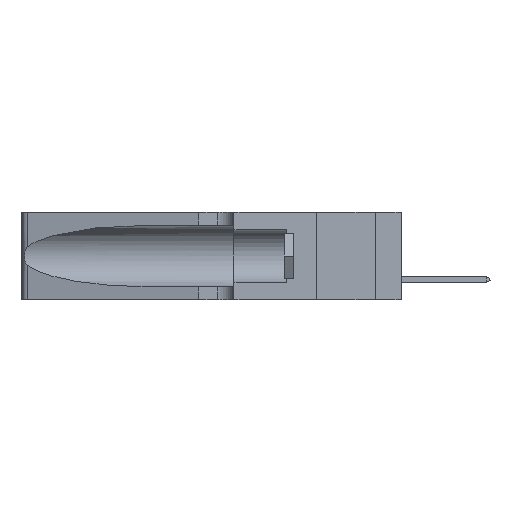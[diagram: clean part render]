
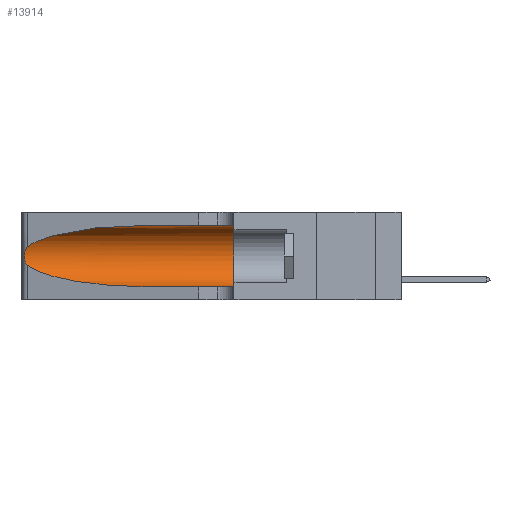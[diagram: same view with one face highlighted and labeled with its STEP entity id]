
A CAD part, left-side view. The second image highlights one B-rep face of the part: STEP entity #13914.
In plain terms, the highlighted cylindrical face has radius 3.308 mm (diameter 6.617 mm), a partial arc.
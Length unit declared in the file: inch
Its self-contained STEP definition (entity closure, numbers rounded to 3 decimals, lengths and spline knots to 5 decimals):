
#699 = DIRECTION ( 'NONE',  ( 0., -1., 0. ) ) ;
#1340 = CARTESIAN_POINT ( 'NONE',  ( 0.25487, 1.22718, 0.22369 ) ) ;
#1748 = ORIENTED_EDGE ( 'NONE', *, *, #21089, .T. ) ;
#2220 = VERTEX_POINT ( 'NONE', #32454 ) ;
#2355 = CARTESIAN_POINT ( 'NONE',  ( 0.1305, 1.61858, 0.05475 ) ) ;
#2359 = CARTESIAN_POINT ( 'NONE',  ( 0.26075, 1.23896, 0.19203 ) ) ;
#2430 = AXIS2_PLACEMENT_3D ( 'NONE', #25510, #30448, #20397 ) ;
#2759 = CARTESIAN_POINT ( 'NONE',  ( 0.1305, 1.61858, 0.31525 ) ) ;
#2851 = VECTOR ( 'NONE', #5037, 39.37008 ) ;
#3721 = EDGE_CURVE ( 'NONE', #10846, #26673, #28995, .T. ) ;
#3957 = DIRECTION ( 'NONE',  ( 0., 0., 1. ) ) ;
#4717 = CARTESIAN_POINT ( 'NONE',  ( 0.25787, 1.23484, 0.2124 ) ) ;
#5037 = DIRECTION ( 'NONE',  ( 0., -1., 0. ) ) ;
#5045 = CARTESIAN_POINT ( 'NONE',  ( 0.25789, 1.23486, 0.15765 ) ) ;
#6165 = CARTESIAN_POINT ( 'NONE',  ( 0.18966, 0.96281, 0.05475 ) ) ;
#7093 = CARTESIAN_POINT ( 'NONE',  ( 0.25487, 1.22718, 0.14631 ) ) ;
#7228 = EDGE_CURVE ( 'NONE', #19252, #17524, #25110, .T. ) ;
#7831 = EDGE_CURVE ( 'NONE', #2220, #19252, #24213, .T. ) ;
#8399 = CARTESIAN_POINT ( 'NONE',  ( 0.2373, 1.15595, 0.08982 ) ) ;
#8485 = CYLINDRICAL_SURFACE ( 'NONE', #2430, 0.13025 ) ;
#9844 = AXIS2_PLACEMENT_3D ( 'NONE', #29628, #32328, #3957 ) ;
#10044 =( BOUNDED_CURVE ( )  B_SPLINE_CURVE ( 3, ( #19012, #8399, #6165, #18335 ),
 .UNSPECIFIED., .F., .T. ) 
 B_SPLINE_CURVE_WITH_KNOTS ( ( 4, 4 ),
 ( 3.44316, 4.71239 ),
 .UNSPECIFIED. ) 
 CURVE ( )  GEOMETRIC_REPRESENTATION_ITEM ( )  RATIONAL_B_SPLINE_CURVE ( ( 1., 0.87, 0.87, 1. ) ) 
 REPRESENTATION_ITEM ( '' )  );
#10526 = CARTESIAN_POINT ( 'NONE',  ( 0.1305, 0.35, 0.05475 ) ) ;
#10846 = VERTEX_POINT ( 'NONE', #13500 ) ;
#11152 = ORIENTED_EDGE ( 'NONE', *, *, #7228, .F. ) ;
#12711 = CARTESIAN_POINT ( 'NONE',  ( 0.25854, 1.2359, 0.20912 ) ) ;
#13500 = CARTESIAN_POINT ( 'NONE',  ( 0.25487, 1.22718, 0.22369 ) ) ;
#13914 = ADVANCED_FACE ( 'NONE', ( #15770 ), #8485, .F. ) ;
#14806 = CARTESIAN_POINT ( 'NONE',  ( 0.25487, 1.22718, 0.14631 ) ) ;
#14880 = CARTESIAN_POINT ( 'NONE',  ( 0.25487, 1.22718, 0.22369 ) ) ;
#15104 = CARTESIAN_POINT ( 'NONE',  ( 0.25639, 1.23186, 0.15144 ) ) ;
#15331 = CARTESIAN_POINT ( 'NONE',  ( 0.26017, 1.23833, 0.17102 ) ) ;
#15755 = ORIENTED_EDGE ( 'NONE', *, *, #7831, .F. ) ;
#15770 = FACE_OUTER_BOUND ( 'NONE', #26112, .T. ) ;
#16399 = CARTESIAN_POINT ( 'NONE',  ( 0.18966, 0.96281, 0.31525 ) ) ;
#16601 = EDGE_CURVE ( 'NONE', #2220, #10846, #22420, .T. ) ;
#17040 = ORIENTED_EDGE ( 'NONE', *, *, #18677, .T. ) ;
#17245 = ORIENTED_EDGE ( 'NONE', *, *, #16601, .T. ) ;
#17480 = CARTESIAN_POINT ( 'NONE',  ( 0.26075, 1.23896, 0.178 ) ) ;
#17524 = VERTEX_POINT ( 'NONE', #10526 ) ;
#18335 = CARTESIAN_POINT ( 'NONE',  ( 0.1305, 0.72297, 0.05475 ) ) ;
#18677 = EDGE_CURVE ( 'NONE', #23108, #17524, #23485, .T. ) ;
#19012 = CARTESIAN_POINT ( 'NONE',  ( 0.25487, 1.22718, 0.14631 ) ) ;
#19252 = VERTEX_POINT ( 'NONE', #24437 ) ;
#20251 = CARTESIAN_POINT ( 'NONE',  ( 0.25856, 1.23593, 0.16098 ) ) ;
#20397 = DIRECTION ( 'NONE',  ( 0., 0., -1. ) ) ;
#21089 = EDGE_CURVE ( 'NONE', #26673, #23108, #10044, .T. ) ;
#21649 = CARTESIAN_POINT ( 'NONE',  ( 0.1305, 0.72297, 0.05475 ) ) ;
#22420 =( BOUNDED_CURVE ( )  B_SPLINE_CURVE ( 3, ( #29225, #16399, #24393, #1340 ),
 .UNSPECIFIED., .F., .T. ) 
 B_SPLINE_CURVE_WITH_KNOTS ( ( 4, 4 ),
 ( 1.5708, 2.84003 ),
 .UNSPECIFIED. ) 
 CURVE ( )  GEOMETRIC_REPRESENTATION_ITEM ( )  RATIONAL_B_SPLINE_CURVE ( ( 1., 0.87, 0.87, 1. ) ) 
 REPRESENTATION_ITEM ( '' )  );
#22715 = CARTESIAN_POINT ( 'NONE',  ( 0.25555, 1.22993, 0.14849 ) ) ;
#23108 = VERTEX_POINT ( 'NONE', #21649 ) ;
#23485 = LINE ( 'NONE', #2355, #31167 ) ;
#24213 = LINE ( 'NONE', #2759, #2851 ) ;
#24393 = CARTESIAN_POINT ( 'NONE',  ( 0.2373, 1.15595, 0.28018 ) ) ;
#24437 = CARTESIAN_POINT ( 'NONE',  ( 0.1305, 0.35, 0.31525 ) ) ;
#24458 = ORIENTED_EDGE ( 'NONE', *, *, #3721, .T. ) ;
#25110 = CIRCLE ( 'NONE', #9844, 0.13025 ) ;
#25510 = CARTESIAN_POINT ( 'NONE',  ( 0.1305, 1.61858, 0.185 ) ) ;
#25566 = CARTESIAN_POINT ( 'NONE',  ( 0.25639, 1.23184, 0.21858 ) ) ;
#26112 = EDGE_LOOP ( 'NONE', ( #17245, #24458, #1748, #17040, #11152, #15755 ) ) ;
#26673 = VERTEX_POINT ( 'NONE', #14806 ) ;
#28123 = CARTESIAN_POINT ( 'NONE',  ( 0.25555, 1.22994, 0.2215 ) ) ;
#28995 = B_SPLINE_CURVE_WITH_KNOTS ( 'NONE', 3,
 ( #14880, #28123, #25566, #4717, #12711, #32862, #2359, #17480, #15331, #20251, #5045, #15104, #22715, #7093 ),
 .UNSPECIFIED., .F., .F.,
 ( 4, 2, 2, 2, 2, 2, 4 ),
 ( 0., 0.00027, 0.00053, 0.00107, 0.0016, 0.00187, 0.00214 ),
 .UNSPECIFIED. ) ;
#29225 = CARTESIAN_POINT ( 'NONE',  ( 0.1305, 0.72297, 0.31525 ) ) ;
#29628 = CARTESIAN_POINT ( 'NONE',  ( 0.1305, 0.35, 0.185 ) ) ;
#30448 = DIRECTION ( 'NONE',  ( 0., -1., 0. ) ) ;
#31167 = VECTOR ( 'NONE', #699, 39.37008 ) ;
#32328 = DIRECTION ( 'NONE',  ( 0., 1., 0. ) ) ;
#32454 = CARTESIAN_POINT ( 'NONE',  ( 0.1305, 0.72297, 0.31525 ) ) ;
#32862 = CARTESIAN_POINT ( 'NONE',  ( 0.26018, 1.23835, 0.19895 ) ) ;
